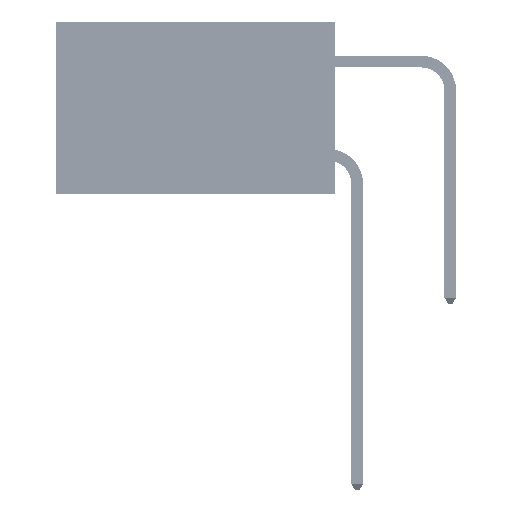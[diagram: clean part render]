
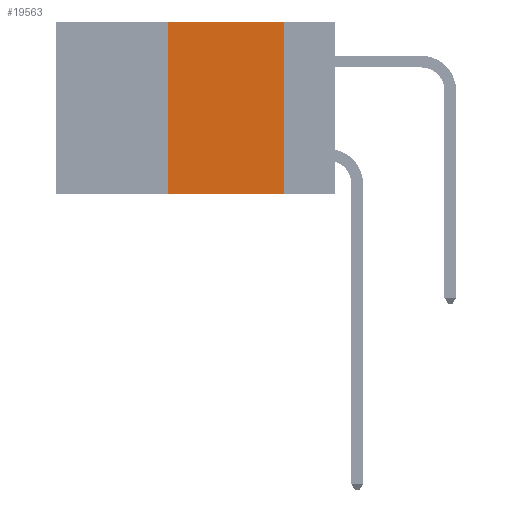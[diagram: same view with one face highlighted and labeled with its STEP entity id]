
A CAD part, left-side view. The second image highlights one B-rep face of the part: STEP entity #19563.
In plain terms, the highlighted planar face has unit normal (-1, 0, 0).
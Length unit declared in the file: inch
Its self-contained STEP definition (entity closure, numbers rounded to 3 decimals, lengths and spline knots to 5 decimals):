
#1058 = PLANE ( 'NONE',  #15398 ) ;
#1209 = VECTOR ( 'NONE', #21123, 39.37008 ) ;
#1650 = VECTOR ( 'NONE', #17277, 39.37008 ) ;
#2929 = DIRECTION ( 'NONE',  ( 0., -1., 0. ) ) ;
#5368 = CARTESIAN_POINT ( 'NONE',  ( 0., 0.36, -0.37 ) ) ;
#5799 = DIRECTION ( 'NONE',  ( 0., -1., 0. ) ) ;
#6016 = LINE ( 'NONE', #37262, #35000 ) ;
#7990 = FACE_OUTER_BOUND ( 'NONE', #8491, .T. ) ;
#8491 = EDGE_LOOP ( 'NONE', ( #46780, #38640, #27063, #12738 ) ) ;
#10089 = LINE ( 'NONE', #32374, #1209 ) ;
#12320 = DIRECTION ( 'NONE',  ( 0., 0., -1. ) ) ;
#12738 = ORIENTED_EDGE ( 'NONE', *, *, #36231, .T. ) ;
#15398 = AXIS2_PLACEMENT_3D ( 'NONE', #16442, #15948, #12320 ) ;
#15948 = DIRECTION ( 'NONE',  ( 1., 0., 0. ) ) ;
#15985 = EDGE_CURVE ( 'NONE', #19749, #21286, #10089, .T. ) ;
#16442 = CARTESIAN_POINT ( 'NONE',  ( 0., 0.6, 0. ) ) ;
#17277 = DIRECTION ( 'NONE',  ( 0., 0., 1. ) ) ;
#19563 = ADVANCED_FACE ( 'NONE', ( #7990 ), #1058, .F. ) ;
#19749 = VERTEX_POINT ( 'NONE', #33998 ) ;
#21123 = DIRECTION ( 'NONE',  ( 0., 0., -1. ) ) ;
#21286 = VERTEX_POINT ( 'NONE', #35475 ) ;
#21592 = CARTESIAN_POINT ( 'NONE',  ( 0., 0.36, 0. ) ) ;
#24712 = CARTESIAN_POINT ( 'NONE',  ( 0., 0.36, 0. ) ) ;
#27063 = ORIENTED_EDGE ( 'NONE', *, *, #43891, .F. ) ;
#32374 = CARTESIAN_POINT ( 'NONE',  ( 0., 0.11, 0. ) ) ;
#33998 = CARTESIAN_POINT ( 'NONE',  ( 0., 0.11, 0. ) ) ;
#35000 = VECTOR ( 'NONE', #2929, 39.37008 ) ;
#35475 = CARTESIAN_POINT ( 'NONE',  ( 0., 0.11, -0.37 ) ) ;
#36231 = EDGE_CURVE ( 'NONE', #41514, #21286, #6016, .T. ) ;
#37056 = VECTOR ( 'NONE', #5799, 39.37008 ) ;
#37262 = CARTESIAN_POINT ( 'NONE',  ( 0., 0.6, -0.37 ) ) ;
#37344 = VERTEX_POINT ( 'NONE', #21592 ) ;
#38640 = ORIENTED_EDGE ( 'NONE', *, *, #44566, .F. ) ;
#39423 = LINE ( 'NONE', #24712, #1650 ) ;
#40095 = CARTESIAN_POINT ( 'NONE',  ( 0., 0.6, 0. ) ) ;
#41514 = VERTEX_POINT ( 'NONE', #5368 ) ;
#43891 = EDGE_CURVE ( 'NONE', #41514, #37344, #39423, .T. ) ;
#44566 = EDGE_CURVE ( 'NONE', #37344, #19749, #44734, .T. ) ;
#44734 = LINE ( 'NONE', #40095, #37056 ) ;
#46780 = ORIENTED_EDGE ( 'NONE', *, *, #15985, .F. ) ;
